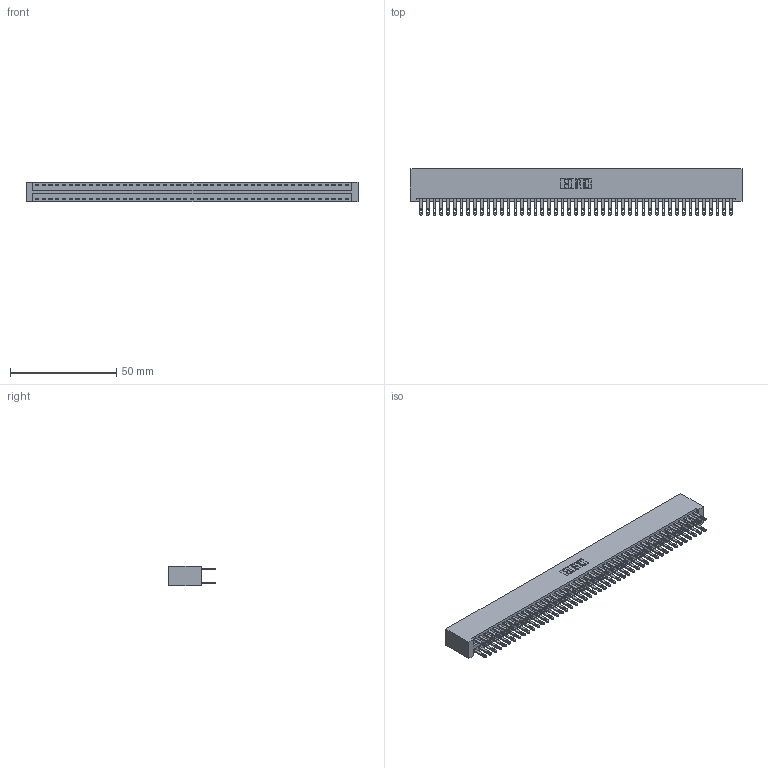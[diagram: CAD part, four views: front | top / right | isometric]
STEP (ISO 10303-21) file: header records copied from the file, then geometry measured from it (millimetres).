
FILE_DESCRIPTION (( 'STEP AP203' ), '1' );
FILE_NAME ('346-094-500-201.STEP', '2022-05-26T09:00:09', ( '' ), ( '' ), 'SwSTEP 2.0', 'SolidWorks 2020', '' );
FILE_SCHEMA (( 'CONFIG_CONTROL_DESIGN' ));
Length unit declared in the file: inch
Products named in the file (3): 345-292-001_345-293-100; 346 Part_No Mounting Lugs; 346-094-500-201
Assembly tree (95 placements, depth 2):
  346-094-500-201
    346 Part_No Mounting Lugs
    345-292-001_345-293-100  x94
Bounding box: 156.46 x 21.84 x 9.4 mm (x, y, z)
Volume: 16156.5 mm3; surface area: 23433.9 mm2
Topology: 95 solids, 95 shells, 4626 faces, 14123 edges, 9414 vertices
Faces by surface type: plane 2798, cylinder 1828
Entity records: 29653 total; most frequent: CARTESIAN_POINT 4876, ORIENTED_EDGE 4810, DIRECTION 4345, EDGE_CURVE 2405, LINE 2089, VECTOR 2089, VERTEX_POINT 1602, AXIS2_PLACEMENT_3D 1128
